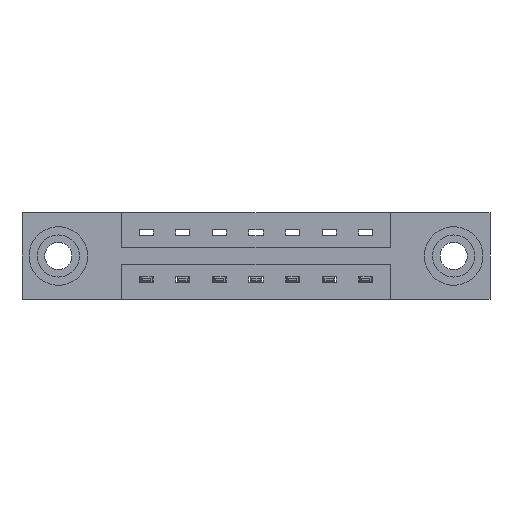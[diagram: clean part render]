
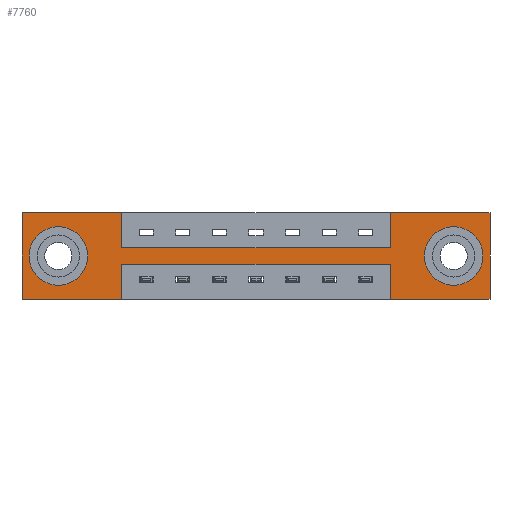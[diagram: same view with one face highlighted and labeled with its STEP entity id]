
A CAD part, front view. The second image highlights one B-rep face of the part: STEP entity #7760.
In plain terms, the highlighted planar face has unit normal (0, -1, 0).
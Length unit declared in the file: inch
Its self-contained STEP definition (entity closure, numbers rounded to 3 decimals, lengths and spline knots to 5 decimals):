
#275 = VERTEX_POINT ( 'NONE', #6036 ) ;
#357 = LINE ( 'NONE', #4642, #10092 ) ;
#361 = CARTESIAN_POINT ( 'NONE',  ( 0.425, 0., -0.37 ) ) ;
#366 = VERTEX_POINT ( 'NONE', #1462 ) ;
#379 = EDGE_CURVE ( 'NONE', #629, #604, #357, .T. ) ;
#399 = CARTESIAN_POINT ( 'NONE',  ( 0., 0., 0. ) ) ;
#462 = EDGE_CURVE ( 'NONE', #1555, #6168, #4168, .T. ) ;
#582 = ORIENTED_EDGE ( 'NONE', *, *, #462, .F. ) ;
#604 = VERTEX_POINT ( 'NONE', #4896 ) ;
#629 = VERTEX_POINT ( 'NONE', #5803 ) ;
#641 = VERTEX_POINT ( 'NONE', #976 ) ;
#734 = EDGE_CURVE ( 'NONE', #641, #7870, #5404, .T. ) ;
#749 = EDGE_CURVE ( 'NONE', #4569, #641, #9964, .T. ) ;
#813 = EDGE_CURVE ( 'NONE', #1911, #1464, #8375, .T. ) ;
#904 = CARTESIAN_POINT ( 'NONE',  ( 1.573, 0., -0.22 ) ) ;
#920 = ORIENTED_EDGE ( 'NONE', *, *, #6534, .T. ) ;
#953 = DIRECTION ( 'NONE',  ( 0., 1., 0. ) ) ;
#976 = CARTESIAN_POINT ( 'NONE',  ( 0.425, 0., -0.22 ) ) ;
#1231 = CARTESIAN_POINT ( 'NONE',  ( 0., 0., 0. ) ) ;
#1292 = AXIS2_PLACEMENT_3D ( 'NONE', #8583, #5561, #4084 ) ;
#1339 = AXIS2_PLACEMENT_3D ( 'NONE', #9749, #9640, #7322 ) ;
#1401 = CARTESIAN_POINT ( 'NONE',  ( 0., 0., -0.37 ) ) ;
#1421 = CARTESIAN_POINT ( 'NONE',  ( 1.843, 0., -0.263 ) ) ;
#1439 = VECTOR ( 'NONE', #4451, 39.37008 ) ;
#1462 = CARTESIAN_POINT ( 'NONE',  ( 0.155, 0., -0.263 ) ) ;
#1464 = VERTEX_POINT ( 'NONE', #5664 ) ;
#1555 = VERTEX_POINT ( 'NONE', #399 ) ;
#1602 = DIRECTION ( 'NONE',  ( 0., 0., -1. ) ) ;
#1707 = CARTESIAN_POINT ( 'NONE',  ( 1.843, 0., -0.185 ) ) ;
#1911 = VERTEX_POINT ( 'NONE', #3612 ) ;
#1962 = EDGE_CURVE ( 'NONE', #6168, #1911, #9471, .T. ) ;
#2049 = CARTESIAN_POINT ( 'NONE',  ( 0.155, 0., -0.185 ) ) ;
#2080 = CARTESIAN_POINT ( 'NONE',  ( 0., 0., -0.37 ) ) ;
#2382 = EDGE_CURVE ( 'NONE', #604, #9000, #8962, .T. ) ;
#2482 = VECTOR ( 'NONE', #6802, 39.37008 ) ;
#2574 = ORIENTED_EDGE ( 'NONE', *, *, #5590, .F. ) ;
#2619 = VECTOR ( 'NONE', #8560, 39.37008 ) ;
#2758 = ORIENTED_EDGE ( 'NONE', *, *, #4705, .T. ) ;
#2812 = ORIENTED_EDGE ( 'NONE', *, *, #749, .F. ) ;
#2922 = LINE ( 'NONE', #2080, #1439 ) ;
#2981 = EDGE_LOOP ( 'NONE', ( #3344, #2812, #4190, #9558, #6346, #4205, #10089, #6206, #9304, #582, #4833, #2574 ) ) ;
#3344 = ORIENTED_EDGE ( 'NONE', *, *, #734, .F. ) ;
#3362 = EDGE_CURVE ( 'NONE', #275, #1555, #4492, .T. ) ;
#3386 = VECTOR ( 'NONE', #3669, 39.37008 ) ;
#3612 = CARTESIAN_POINT ( 'NONE',  ( 0.425, 0., -0.15 ) ) ;
#3669 = DIRECTION ( 'NONE',  ( 0., 0., -1. ) ) ;
#3845 = VERTEX_POINT ( 'NONE', #4843 ) ;
#3887 = CARTESIAN_POINT ( 'NONE',  ( 0.425, 0., -0.15 ) ) ;
#4000 = FACE_BOUND ( 'NONE', #7343, .T. ) ;
#4069 = CARTESIAN_POINT ( 'NONE',  ( 1.843, 0., -0.107 ) ) ;
#4084 = DIRECTION ( 'NONE',  ( 0., 0., 1. ) ) ;
#4160 = VECTOR ( 'NONE', #9464, 39.37008 ) ;
#4168 = LINE ( 'NONE', #6363, #6518 ) ;
#4190 = ORIENTED_EDGE ( 'NONE', *, *, #5234, .F. ) ;
#4205 = ORIENTED_EDGE ( 'NONE', *, *, #379, .F. ) ;
#4208 = AXIS2_PLACEMENT_3D ( 'NONE', #2049, #9879, #5146 ) ;
#4313 = EDGE_CURVE ( 'NONE', #9000, #3845, #9048, .T. ) ;
#4319 = CARTESIAN_POINT ( 'NONE',  ( 0.425, 0., -0.22 ) ) ;
#4438 = VERTEX_POINT ( 'NONE', #5402 ) ;
#4451 = DIRECTION ( 'NONE',  ( -1., 0., 0. ) ) ;
#4492 = LINE ( 'NONE', #1231, #6849 ) ;
#4569 = VERTEX_POINT ( 'NONE', #904 ) ;
#4642 = CARTESIAN_POINT ( 'NONE',  ( 0., 0., 0. ) ) ;
#4705 = EDGE_CURVE ( 'NONE', #8305, #10013, #5916, .T. ) ;
#4833 = ORIENTED_EDGE ( 'NONE', *, *, #3362, .F. ) ;
#4843 = CARTESIAN_POINT ( 'NONE',  ( 1.573, 0., -0.37 ) ) ;
#4896 = CARTESIAN_POINT ( 'NONE',  ( 1.998, 0., 0. ) ) ;
#5112 = DIRECTION ( 'NONE',  ( 0., 0., -1. ) ) ;
#5146 = DIRECTION ( 'NONE',  ( 0., 0., 1. ) ) ;
#5205 = CIRCLE ( 'NONE', #4208, 0.078 ) ;
#5230 = CARTESIAN_POINT ( 'NONE',  ( 0.425, 0., 0. ) ) ;
#5234 = EDGE_CURVE ( 'NONE', #3845, #4569, #5399, .T. ) ;
#5399 = LINE ( 'NONE', #6330, #4160 ) ;
#5402 = CARTESIAN_POINT ( 'NONE',  ( 0.155, 0., -0.107 ) ) ;
#5404 = LINE ( 'NONE', #361, #6155 ) ;
#5473 = DIRECTION ( 'NONE',  ( 1., 0., 0. ) ) ;
#5513 = AXIS2_PLACEMENT_3D ( 'NONE', #1401, #7729, #6043 ) ;
#5561 = DIRECTION ( 'NONE',  ( 0., 1., 0. ) ) ;
#5590 = EDGE_CURVE ( 'NONE', #7870, #275, #2922, .T. ) ;
#5592 = CIRCLE ( 'NONE', #1292, 0.078 ) ;
#5629 = DIRECTION ( 'NONE',  ( 1., 0., 0. ) ) ;
#5664 = CARTESIAN_POINT ( 'NONE',  ( 1.573, 0., -0.15 ) ) ;
#5803 = CARTESIAN_POINT ( 'NONE',  ( 1.573, 0., 0. ) ) ;
#5916 = CIRCLE ( 'NONE', #1339, 0.078 ) ;
#6036 = CARTESIAN_POINT ( 'NONE',  ( 0., 0., -0.37 ) ) ;
#6037 = CARTESIAN_POINT ( 'NONE',  ( 1.998, 0., -0.37 ) ) ;
#6043 = DIRECTION ( 'NONE',  ( 0., 0., -1. ) ) ;
#6102 = DIRECTION ( 'NONE',  ( 0., 0., -1. ) ) ;
#6155 = VECTOR ( 'NONE', #5112, 39.37008 ) ;
#6168 = VERTEX_POINT ( 'NONE', #7544 ) ;
#6206 = ORIENTED_EDGE ( 'NONE', *, *, #813, .F. ) ;
#6237 = FACE_OUTER_BOUND ( 'NONE', #2981, .T. ) ;
#6330 = CARTESIAN_POINT ( 'NONE',  ( 1.573, 0., -0.37 ) ) ;
#6346 = ORIENTED_EDGE ( 'NONE', *, *, #2382, .F. ) ;
#6363 = CARTESIAN_POINT ( 'NONE',  ( 0., 0., 0. ) ) ;
#6518 = VECTOR ( 'NONE', #5629, 39.37008 ) ;
#6534 = EDGE_CURVE ( 'NONE', #10013, #8305, #10074, .T. ) ;
#6535 = ORIENTED_EDGE ( 'NONE', *, *, #9141, .T. ) ;
#6802 = DIRECTION ( 'NONE',  ( -1., 0., 0. ) ) ;
#6849 = VECTOR ( 'NONE', #9961, 39.37008 ) ;
#6900 = VECTOR ( 'NONE', #5473, 39.37008 ) ;
#7256 = AXIS2_PLACEMENT_3D ( 'NONE', #1707, #953, #1602 ) ;
#7301 = ORIENTED_EDGE ( 'NONE', *, *, #7903, .T. ) ;
#7311 = DIRECTION ( 'NONE',  ( 1., 0., 0. ) ) ;
#7322 = DIRECTION ( 'NONE',  ( 0., 0., -1. ) ) ;
#7343 = EDGE_LOOP ( 'NONE', ( #2758, #920 ) ) ;
#7395 = VECTOR ( 'NONE', #6102, 39.37008 ) ;
#7521 = VECTOR ( 'NONE', #9809, 39.37008 ) ;
#7544 = CARTESIAN_POINT ( 'NONE',  ( 0.425, 0., 0. ) ) ;
#7729 = DIRECTION ( 'NONE',  ( 0., -1., 0. ) ) ;
#7760 = ADVANCED_FACE ( 'NONE', ( #4000, #8340, #6237 ), #10026, .T. ) ;
#7870 = VERTEX_POINT ( 'NONE', #10156 ) ;
#7903 = EDGE_CURVE ( 'NONE', #4438, #366, #5592, .T. ) ;
#8305 = VERTEX_POINT ( 'NONE', #4069 ) ;
#8340 = FACE_BOUND ( 'NONE', #8509, .T. ) ;
#8375 = LINE ( 'NONE', #3887, #6900 ) ;
#8509 = EDGE_LOOP ( 'NONE', ( #7301, #6535 ) ) ;
#8560 = DIRECTION ( 'NONE',  ( 0., 0., 1. ) ) ;
#8583 = CARTESIAN_POINT ( 'NONE',  ( 0.155, 0., -0.185 ) ) ;
#8688 = EDGE_CURVE ( 'NONE', #1464, #629, #9177, .T. ) ;
#8962 = LINE ( 'NONE', #8992, #3386 ) ;
#8992 = CARTESIAN_POINT ( 'NONE',  ( 1.998, 0., 0. ) ) ;
#9000 = VERTEX_POINT ( 'NONE', #6037 ) ;
#9048 = LINE ( 'NONE', #9237, #2482 ) ;
#9141 = EDGE_CURVE ( 'NONE', #366, #4438, #5205, .T. ) ;
#9177 = LINE ( 'NONE', #10098, #2619 ) ;
#9237 = CARTESIAN_POINT ( 'NONE',  ( 0., 0., -0.37 ) ) ;
#9304 = ORIENTED_EDGE ( 'NONE', *, *, #1962, .F. ) ;
#9464 = DIRECTION ( 'NONE',  ( 0., 0., 1. ) ) ;
#9471 = LINE ( 'NONE', #5230, #7395 ) ;
#9558 = ORIENTED_EDGE ( 'NONE', *, *, #4313, .F. ) ;
#9640 = DIRECTION ( 'NONE',  ( 0., 1., 0. ) ) ;
#9749 = CARTESIAN_POINT ( 'NONE',  ( 1.843, 0., -0.185 ) ) ;
#9809 = DIRECTION ( 'NONE',  ( -1., 0., 0. ) ) ;
#9879 = DIRECTION ( 'NONE',  ( 0., 1., 0. ) ) ;
#9961 = DIRECTION ( 'NONE',  ( 0., 0., 1. ) ) ;
#9964 = LINE ( 'NONE', #4319, #7521 ) ;
#10013 = VERTEX_POINT ( 'NONE', #1421 ) ;
#10026 = PLANE ( 'NONE',  #5513 ) ;
#10074 = CIRCLE ( 'NONE', #7256, 0.078 ) ;
#10089 = ORIENTED_EDGE ( 'NONE', *, *, #8688, .F. ) ;
#10092 = VECTOR ( 'NONE', #7311, 39.37008 ) ;
#10098 = CARTESIAN_POINT ( 'NONE',  ( 1.573, 0., 0. ) ) ;
#10156 = CARTESIAN_POINT ( 'NONE',  ( 0.425, 0., -0.37 ) ) ;
